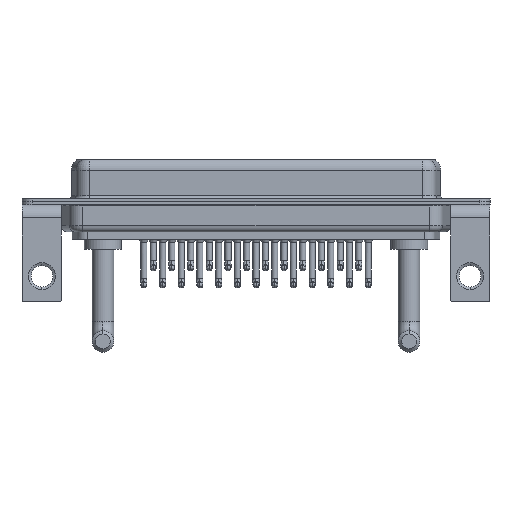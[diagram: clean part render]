
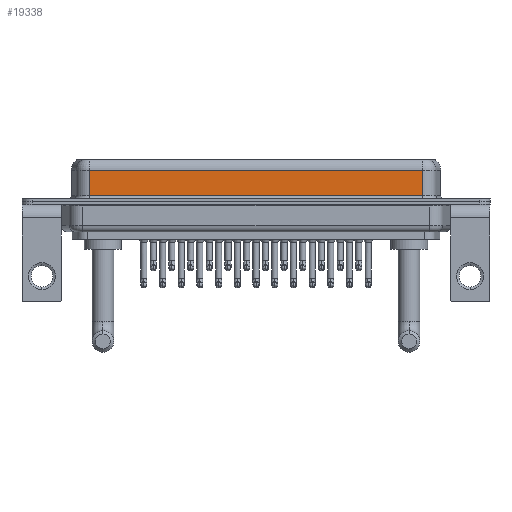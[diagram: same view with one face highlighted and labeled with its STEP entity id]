
A CAD part, front view. The second image highlights one B-rep face of the part: STEP entity #19338.
In plain terms, the highlighted planar face has unit normal (0, -1, 0).
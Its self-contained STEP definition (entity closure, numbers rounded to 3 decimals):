
#490 = VECTOR ( 'NONE', #3347, 1000. ) ;
#1155 = CARTESIAN_POINT ( 'NONE',  ( 7.038, -3.95, 6.4 ) ) ;
#1352 = AXIS2_PLACEMENT_3D ( 'NONE', #11838, #15622, #2151 ) ;
#2151 = DIRECTION ( 'NONE',  ( 0., 0., 1. ) ) ;
#3347 = DIRECTION ( 'NONE',  ( 0., 0., -1. ) ) ;
#3869 = CARTESIAN_POINT ( 'NONE',  ( 56.462, -3.95, 6.4 ) ) ;
#5825 = DIRECTION ( 'NONE',  ( -1., 0., 0. ) ) ;
#6288 = EDGE_CURVE ( 'NONE', #23714, #18789, #21089, .T. ) ;
#6368 = ORIENTED_EDGE ( 'NONE', *, *, #14949, .T. ) ;
#7750 = LINE ( 'NONE', #3869, #11447 ) ;
#8048 = VECTOR ( 'NONE', #17529, 1000. ) ;
#8285 = ORIENTED_EDGE ( 'NONE', *, *, #6288, .T. ) ;
#8805 = CARTESIAN_POINT ( 'NONE',  ( 7.038, -3.95, 0.9 ) ) ;
#9041 = ORIENTED_EDGE ( 'NONE', *, *, #25279, .F. ) ;
#9725 = LINE ( 'NONE', #21901, #8048 ) ;
#11073 = CARTESIAN_POINT ( 'NONE',  ( 56.462, -3.95, 0.9 ) ) ;
#11171 = CARTESIAN_POINT ( 'NONE',  ( 56.462, -3.95, 4.65 ) ) ;
#11447 = VECTOR ( 'NONE', #25480, 1000. ) ;
#11838 = CARTESIAN_POINT ( 'NONE',  ( 56.462, -3.95, 6.4 ) ) ;
#14949 = EDGE_CURVE ( 'NONE', #18789, #17714, #9725, .T. ) ;
#15035 = EDGE_CURVE ( 'NONE', #22891, #23714, #21516, .T. ) ;
#15622 = DIRECTION ( 'NONE',  ( 0., 1., 0. ) ) ;
#15748 = PLANE ( 'NONE',  #1352 ) ;
#15811 = CARTESIAN_POINT ( 'NONE',  ( 7.038, -3.95, 4.65 ) ) ;
#17323 = FACE_OUTER_BOUND ( 'NONE', #17403, .T. ) ;
#17395 = CARTESIAN_POINT ( 'NONE',  ( 56.462, -3.95, 4.65 ) ) ;
#17403 = EDGE_LOOP ( 'NONE', ( #9041, #23256, #8285, #6368 ) ) ;
#17529 = DIRECTION ( 'NONE',  ( 1., 0., 0. ) ) ;
#17714 = VERTEX_POINT ( 'NONE', #11073 ) ;
#18789 = VERTEX_POINT ( 'NONE', #8805 ) ;
#19338 = ADVANCED_FACE ( 'NONE', ( #17323 ), #15748, .F. ) ;
#20855 = VECTOR ( 'NONE', #5825, 1000. ) ;
#21089 = LINE ( 'NONE', #1155, #490 ) ;
#21516 = LINE ( 'NONE', #17395, #20855 ) ;
#21901 = CARTESIAN_POINT ( 'NONE',  ( 56.462, -3.95, 0.9 ) ) ;
#22891 = VERTEX_POINT ( 'NONE', #11171 ) ;
#23256 = ORIENTED_EDGE ( 'NONE', *, *, #15035, .T. ) ;
#23714 = VERTEX_POINT ( 'NONE', #15811 ) ;
#25279 = EDGE_CURVE ( 'NONE', #22891, #17714, #7750, .T. ) ;
#25480 = DIRECTION ( 'NONE',  ( 0., 0., -1. ) ) ;
